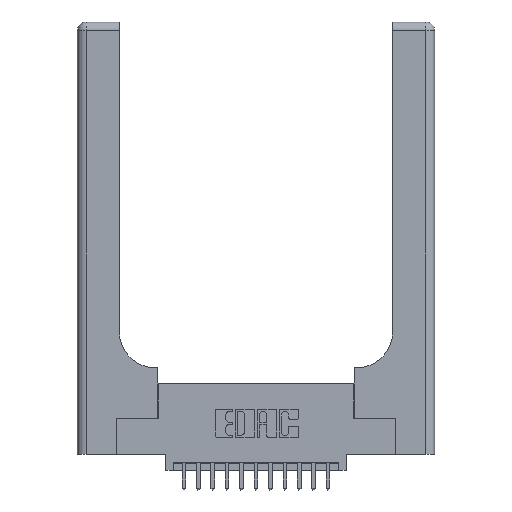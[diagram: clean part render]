
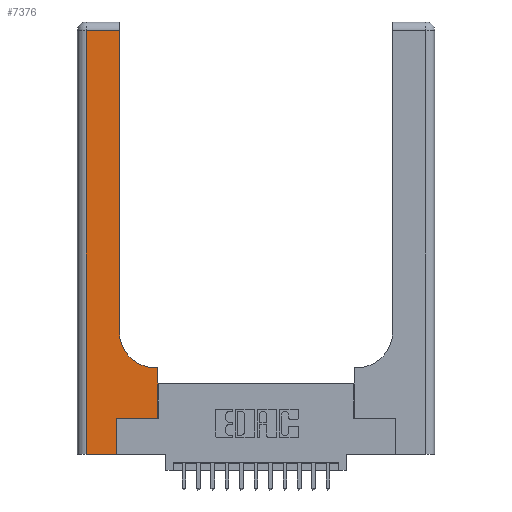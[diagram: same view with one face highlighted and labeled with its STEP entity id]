
A CAD part, top view. The second image highlights one B-rep face of the part: STEP entity #7376.
In plain terms, the highlighted planar face has unit normal (0, 0, 1).
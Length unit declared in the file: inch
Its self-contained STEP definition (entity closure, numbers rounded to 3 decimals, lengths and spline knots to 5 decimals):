
#28 = CARTESIAN_POINT ( 'NONE',  ( 0., 0., 0.37 ) ) ;
#251 = LINE ( 'NONE', #11675, #9281 ) ;
#855 = DIRECTION ( 'NONE',  ( 0., 0., -1. ) ) ;
#954 = CARTESIAN_POINT ( 'NONE',  ( 0.2915, 0.85, 0.37 ) ) ;
#959 = CARTESIAN_POINT ( 'NONE',  ( 0.2915, 2.94, 0.37 ) ) ;
#1188 = DIRECTION ( 'NONE',  ( 1., 0., 0. ) ) ;
#1632 = ORIENTED_EDGE ( 'NONE', *, *, #8146, .T. ) ;
#1757 = VERTEX_POINT ( 'NONE', #11472 ) ;
#2072 = LINE ( 'NONE', #17506, #17011 ) ;
#2200 = DIRECTION ( 'NONE',  ( 0., 1., 0. ) ) ;
#2521 = CARTESIAN_POINT ( 'NONE',  ( 0.06, 2.94, 0.37 ) ) ;
#2668 = EDGE_CURVE ( 'NONE', #1757, #8969, #251, .T. ) ;
#2750 = EDGE_CURVE ( 'NONE', #10852, #7541, #7280, .T. ) ;
#2964 = EDGE_CURVE ( 'NONE', #11674, #3067, #11883, .T. ) ;
#3067 = VERTEX_POINT ( 'NONE', #17323 ) ;
#3286 = EDGE_CURVE ( 'NONE', #11892, #11674, #3293, .T. ) ;
#3293 = LINE ( 'NONE', #28, #11428 ) ;
#3312 = DIRECTION ( 'NONE',  ( 0., 1., 0. ) ) ;
#3627 = LINE ( 'NONE', #11579, #6710 ) ;
#3675 = CARTESIAN_POINT ( 'NONE',  ( 0.269, 0., 0.37 ) ) ;
#3756 = VECTOR ( 'NONE', #2200, 39.37008 ) ;
#3815 = ORIENTED_EDGE ( 'NONE', *, *, #2964, .T. ) ;
#4267 = VERTEX_POINT ( 'NONE', #2521 ) ;
#4344 = VERTEX_POINT ( 'NONE', #959 ) ;
#4545 = PLANE ( 'NONE',  #12039 ) ;
#5301 = CARTESIAN_POINT ( 'NONE',  ( 0.269, 0., 0.37 ) ) ;
#5540 = ORIENTED_EDGE ( 'NONE', *, *, #10664, .T. ) ;
#5752 = ORIENTED_EDGE ( 'NONE', *, *, #9118, .T. ) ;
#6250 = DIRECTION ( 'NONE',  ( 0., 1., 0. ) ) ;
#6356 = CARTESIAN_POINT ( 'NONE',  ( 0., 3., 0.37 ) ) ;
#6610 = DIRECTION ( 'NONE',  ( 1., 0., 0. ) ) ;
#6710 = VECTOR ( 'NONE', #7184, 39.37008 ) ;
#6941 = CARTESIAN_POINT ( 'NONE',  ( 0.269, 0.25, 0.37 ) ) ;
#7118 = VECTOR ( 'NONE', #6250, 39.37008 ) ;
#7184 = DIRECTION ( 'NONE',  ( -1., 0., 0. ) ) ;
#7280 = CIRCLE ( 'NONE', #12923, 0.25 ) ;
#7376 = ADVANCED_FACE ( 'NONE', ( #15892 ), #4545, .F. ) ;
#7541 = VERTEX_POINT ( 'NONE', #954 ) ;
#7852 = DIRECTION ( 'NONE',  ( -1., 0., 0. ) ) ;
#8146 = EDGE_CURVE ( 'NONE', #3067, #1757, #14316, .T. ) ;
#8898 = ORIENTED_EDGE ( 'NONE', *, *, #2668, .T. ) ;
#8969 = VERTEX_POINT ( 'NONE', #14962 ) ;
#9118 = EDGE_CURVE ( 'NONE', #8969, #10852, #3627, .T. ) ;
#9281 = VECTOR ( 'NONE', #3312, 39.37008 ) ;
#10140 = EDGE_CURVE ( 'NONE', #4267, #11892, #2072, .T. ) ;
#10423 = ORIENTED_EDGE ( 'NONE', *, *, #13946, .T. ) ;
#10664 = EDGE_CURVE ( 'NONE', #7541, #4344, #13690, .T. ) ;
#10752 = VECTOR ( 'NONE', #17426, 39.37008 ) ;
#10852 = VERTEX_POINT ( 'NONE', #17544 ) ;
#10964 = DIRECTION ( 'NONE',  ( 0., 0., -1. ) ) ;
#11428 = VECTOR ( 'NONE', #6610, 39.37008 ) ;
#11472 = CARTESIAN_POINT ( 'NONE',  ( 0.5585, 0.25, 0.37 ) ) ;
#11579 = CARTESIAN_POINT ( 'NONE',  ( 0.2915, 0.6, 0.37 ) ) ;
#11674 = VERTEX_POINT ( 'NONE', #5301 ) ;
#11675 = CARTESIAN_POINT ( 'NONE',  ( 0.5585, 0.25, 0.37 ) ) ;
#11759 = CARTESIAN_POINT ( 'NONE',  ( 0., 2.94, 0.37 ) ) ;
#11883 = LINE ( 'NONE', #3675, #3756 ) ;
#11892 = VERTEX_POINT ( 'NONE', #17203 ) ;
#12008 = ORIENTED_EDGE ( 'NONE', *, *, #3286, .T. ) ;
#12039 = AXIS2_PLACEMENT_3D ( 'NONE', #6356, #855, #7852 ) ;
#12071 = LINE ( 'NONE', #11759, #10752 ) ;
#12643 = ORIENTED_EDGE ( 'NONE', *, *, #10140, .T. ) ;
#12923 = AXIS2_PLACEMENT_3D ( 'NONE', #15177, #10964, #1188 ) ;
#13690 = LINE ( 'NONE', #15952, #7118 ) ;
#13946 = EDGE_CURVE ( 'NONE', #4344, #4267, #12071, .T. ) ;
#14316 = LINE ( 'NONE', #6941, #14560 ) ;
#14560 = VECTOR ( 'NONE', #17782, 39.37008 ) ;
#14567 = ORIENTED_EDGE ( 'NONE', *, *, #2750, .T. ) ;
#14962 = CARTESIAN_POINT ( 'NONE',  ( 0.5585, 0.6, 0.37 ) ) ;
#15177 = CARTESIAN_POINT ( 'NONE',  ( 0.5415, 0.85, 0.37 ) ) ;
#15320 = EDGE_LOOP ( 'NONE', ( #5540, #10423, #12643, #12008, #3815, #1632, #8898, #5752, #14567 ) ) ;
#15892 = FACE_OUTER_BOUND ( 'NONE', #15320, .T. ) ;
#15952 = CARTESIAN_POINT ( 'NONE',  ( 0.2915, 3., 0.37 ) ) ;
#17011 = VECTOR ( 'NONE', #17439, 39.37008 ) ;
#17203 = CARTESIAN_POINT ( 'NONE',  ( 0.06, 0., 0.37 ) ) ;
#17323 = CARTESIAN_POINT ( 'NONE',  ( 0.269, 0.25, 0.37 ) ) ;
#17426 = DIRECTION ( 'NONE',  ( -1., 0., 0. ) ) ;
#17439 = DIRECTION ( 'NONE',  ( 0., -1., 0. ) ) ;
#17506 = CARTESIAN_POINT ( 'NONE',  ( 0.06, 3., 0.37 ) ) ;
#17544 = CARTESIAN_POINT ( 'NONE',  ( 0.5415, 0.6, 0.37 ) ) ;
#17782 = DIRECTION ( 'NONE',  ( 1., 0., 0. ) ) ;
